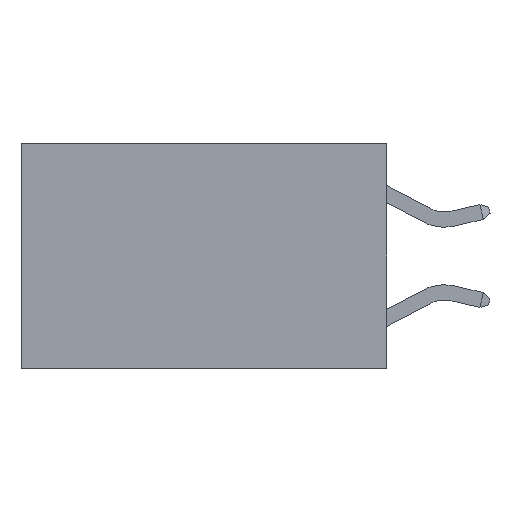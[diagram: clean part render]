
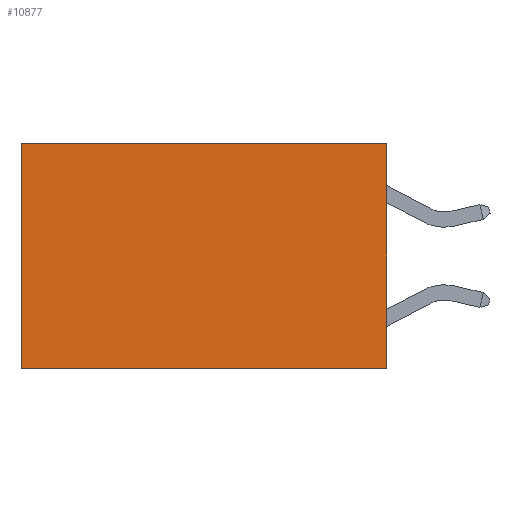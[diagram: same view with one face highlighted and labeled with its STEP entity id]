
A CAD part, left-side view. The second image highlights one B-rep face of the part: STEP entity #10877.
In plain terms, the highlighted planar face has unit normal (-1, 0, 0).
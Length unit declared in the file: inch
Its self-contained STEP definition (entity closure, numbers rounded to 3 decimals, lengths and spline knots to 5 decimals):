
#642 = CARTESIAN_POINT ( 'NONE',  ( 0.2625, 0., -0.37 ) ) ;
#1346 = VERTEX_POINT ( 'NONE', #2412 ) ;
#2095 = CARTESIAN_POINT ( 'NONE',  ( 0.2625, 0., 0. ) ) ;
#2412 = CARTESIAN_POINT ( 'NONE',  ( 0.2625, 0.6, -0.37 ) ) ;
#2504 = CARTESIAN_POINT ( 'NONE',  ( 0.2625, 0., 0. ) ) ;
#3285 = VERTEX_POINT ( 'NONE', #7798 ) ;
#4013 = DIRECTION ( 'NONE',  ( 0., 0., -1. ) ) ;
#5642 = CARTESIAN_POINT ( 'NONE',  ( 0.2625, 0., 0. ) ) ;
#5743 = ORIENTED_EDGE ( 'NONE', *, *, #9767, .F. ) ;
#6223 = ORIENTED_EDGE ( 'NONE', *, *, #10837, .T. ) ;
#6881 = CARTESIAN_POINT ( 'NONE',  ( 0.2625, 0., 0. ) ) ;
#6915 = DIRECTION ( 'NONE',  ( 0., 0., -1. ) ) ;
#7136 = DIRECTION ( 'NONE',  ( 0., 0., -1. ) ) ;
#7798 = CARTESIAN_POINT ( 'NONE',  ( 0.2625, 0.6, 0. ) ) ;
#8416 = PLANE ( 'NONE',  #18127 ) ;
#8693 = LINE ( 'NONE', #5642, #16008 ) ;
#9159 = VECTOR ( 'NONE', #18945, 39.37008 ) ;
#9519 = DIRECTION ( 'NONE',  ( 0., 1., 0. ) ) ;
#9767 = EDGE_CURVE ( 'NONE', #18660, #1346, #13055, .T. ) ;
#9992 = EDGE_LOOP ( 'NONE', ( #13909, #5743, #14789, #6223 ) ) ;
#10246 = VECTOR ( 'NONE', #9519, 39.37008 ) ;
#10837 = EDGE_CURVE ( 'NONE', #15513, #3285, #14600, .T. ) ;
#10877 = ADVANCED_FACE ( 'NONE', ( #13230 ), #8416, .F. ) ;
#12844 = DIRECTION ( 'NONE',  ( 1., 0., 0. ) ) ;
#13055 = LINE ( 'NONE', #17491, #9159 ) ;
#13230 = FACE_OUTER_BOUND ( 'NONE', #9992, .T. ) ;
#13909 = ORIENTED_EDGE ( 'NONE', *, *, #14788, .T. ) ;
#14200 = CARTESIAN_POINT ( 'NONE',  ( 0.2625, 0.6, 0. ) ) ;
#14600 = LINE ( 'NONE', #2095, #10246 ) ;
#14788 = EDGE_CURVE ( 'NONE', #3285, #1346, #19045, .T. ) ;
#14789 = ORIENTED_EDGE ( 'NONE', *, *, #17557, .F. ) ;
#15513 = VERTEX_POINT ( 'NONE', #6881 ) ;
#15613 = VECTOR ( 'NONE', #6915, 39.37008 ) ;
#16008 = VECTOR ( 'NONE', #7136, 39.37008 ) ;
#17491 = CARTESIAN_POINT ( 'NONE',  ( 0.2625, 0., -0.37 ) ) ;
#17557 = EDGE_CURVE ( 'NONE', #15513, #18660, #8693, .T. ) ;
#18127 = AXIS2_PLACEMENT_3D ( 'NONE', #2504, #12844, #4013 ) ;
#18660 = VERTEX_POINT ( 'NONE', #642 ) ;
#18945 = DIRECTION ( 'NONE',  ( 0., 1., 0. ) ) ;
#19045 = LINE ( 'NONE', #14200, #15613 ) ;
